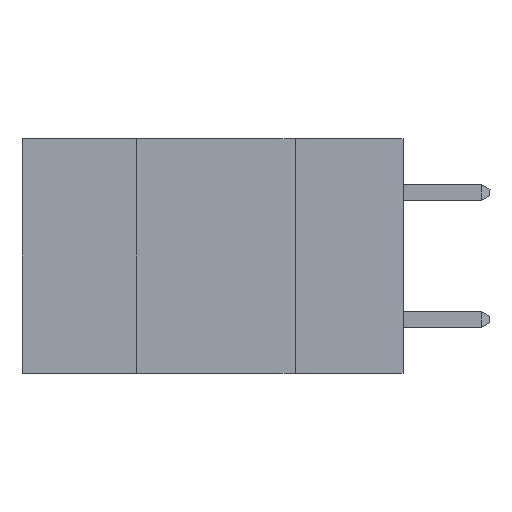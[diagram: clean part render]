
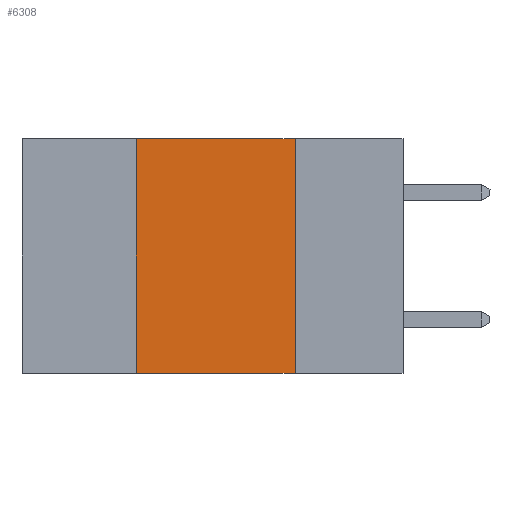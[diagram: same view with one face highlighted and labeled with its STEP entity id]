
A CAD part, left-side view. The second image highlights one B-rep face of the part: STEP entity #6308.
In plain terms, the highlighted planar face has unit normal (-1, 0, 0).
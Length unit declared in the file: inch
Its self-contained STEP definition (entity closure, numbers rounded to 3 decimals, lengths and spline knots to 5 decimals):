
#518 = VERTEX_POINT ( 'NONE', #6356 ) ;
#812 = DIRECTION ( 'NONE',  ( 1., 0., 0. ) ) ;
#881 = CARTESIAN_POINT ( 'NONE',  ( 0., 0.17, 0. ) ) ;
#967 = EDGE_CURVE ( 'NONE', #12875, #518, #12547, .T. ) ;
#1213 = CARTESIAN_POINT ( 'NONE',  ( 0., 0.42, 0. ) ) ;
#1780 = EDGE_CURVE ( 'NONE', #12875, #10229, #7311, .T. ) ;
#2420 = CARTESIAN_POINT ( 'NONE',  ( 0., 0.17, 0. ) ) ;
#2757 = DIRECTION ( 'NONE',  ( 0., -1., 0. ) ) ;
#2895 = VECTOR ( 'NONE', #2757, 39.37008 ) ;
#3200 = PLANE ( 'NONE',  #13156 ) ;
#3524 = EDGE_LOOP ( 'NONE', ( #5770, #6135, #6152, #6855 ) ) ;
#4013 = VECTOR ( 'NONE', #6260, 39.37008 ) ;
#4385 = CARTESIAN_POINT ( 'NONE',  ( 0., 0.42, -0.37 ) ) ;
#4419 = EDGE_CURVE ( 'NONE', #7792, #518, #8751, .T. ) ;
#5770 = ORIENTED_EDGE ( 'NONE', *, *, #4419, .F. ) ;
#6083 = CARTESIAN_POINT ( 'NONE',  ( 0., 0.6, 0. ) ) ;
#6135 = ORIENTED_EDGE ( 'NONE', *, *, #9084, .F. ) ;
#6152 = ORIENTED_EDGE ( 'NONE', *, *, #1780, .F. ) ;
#6260 = DIRECTION ( 'NONE',  ( 0., 0., 1. ) ) ;
#6308 = ADVANCED_FACE ( 'NONE', ( #7923 ), #3200, .F. ) ;
#6356 = CARTESIAN_POINT ( 'NONE',  ( 0., 0.17, -0.37 ) ) ;
#6374 = CARTESIAN_POINT ( 'NONE',  ( 0., 0.6, -0.37 ) ) ;
#6855 = ORIENTED_EDGE ( 'NONE', *, *, #967, .T. ) ;
#6930 = CARTESIAN_POINT ( 'NONE',  ( 0., 0.42, 0. ) ) ;
#7311 = LINE ( 'NONE', #6930, #4013 ) ;
#7792 = VERTEX_POINT ( 'NONE', #2420 ) ;
#7923 = FACE_OUTER_BOUND ( 'NONE', #3524, .T. ) ;
#8581 = DIRECTION ( 'NONE',  ( 0., -1., 0. ) ) ;
#8751 = LINE ( 'NONE', #881, #11886 ) ;
#9084 = EDGE_CURVE ( 'NONE', #10229, #7792, #13915, .T. ) ;
#9359 = DIRECTION ( 'NONE',  ( 0., 0., -1. ) ) ;
#10229 = VERTEX_POINT ( 'NONE', #1213 ) ;
#10837 = VECTOR ( 'NONE', #8581, 39.37008 ) ;
#11886 = VECTOR ( 'NONE', #12930, 39.37008 ) ;
#12547 = LINE ( 'NONE', #6374, #2895 ) ;
#12875 = VERTEX_POINT ( 'NONE', #4385 ) ;
#12930 = DIRECTION ( 'NONE',  ( 0., 0., -1. ) ) ;
#13156 = AXIS2_PLACEMENT_3D ( 'NONE', #13989, #812, #9359 ) ;
#13915 = LINE ( 'NONE', #6083, #10837 ) ;
#13989 = CARTESIAN_POINT ( 'NONE',  ( 0., 0.6, 0. ) ) ;
